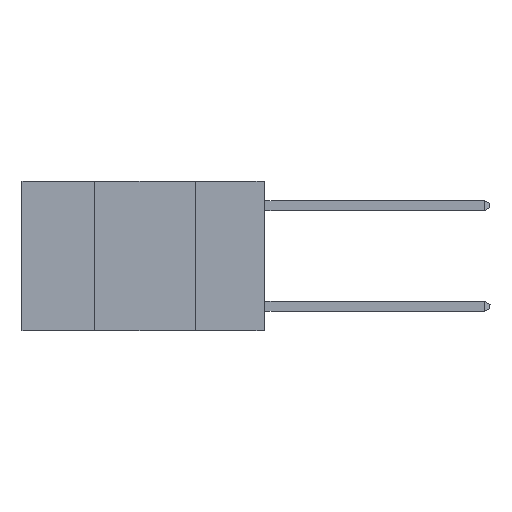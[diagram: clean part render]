
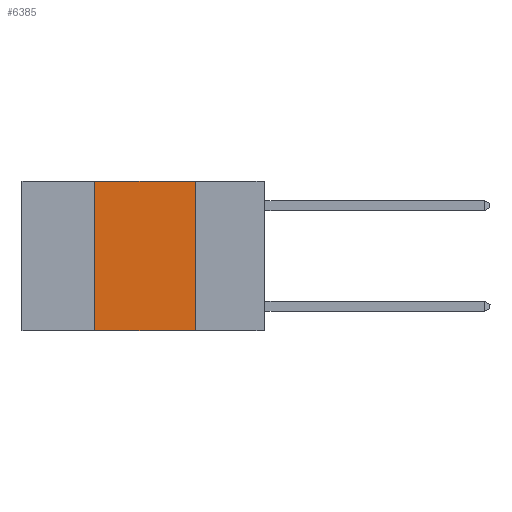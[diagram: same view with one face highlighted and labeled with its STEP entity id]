
A CAD part, left-side view. The second image highlights one B-rep face of the part: STEP entity #6385.
In plain terms, the highlighted planar face has unit normal (-1, 0, 0).
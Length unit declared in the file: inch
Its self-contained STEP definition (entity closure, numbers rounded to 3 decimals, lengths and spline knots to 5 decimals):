
#307 = VECTOR ( 'NONE', #6357, 39.37008 ) ;
#626 = PLANE ( 'NONE',  #1616 ) ;
#719 = LINE ( 'NONE', #3671, #14785 ) ;
#1616 = AXIS2_PLACEMENT_3D ( 'NONE', #10398, #2004, #11815 ) ;
#1763 = CARTESIAN_POINT ( 'NONE',  ( 0., 0.17, 0. ) ) ;
#1870 = VERTEX_POINT ( 'NONE', #9397 ) ;
#2004 = DIRECTION ( 'NONE',  ( 1., 0., 0. ) ) ;
#2241 = DIRECTION ( 'NONE',  ( 0., -1., 0. ) ) ;
#2290 = ORIENTED_EDGE ( 'NONE', *, *, #3329, .F. ) ;
#3329 = EDGE_CURVE ( 'NONE', #8819, #15139, #15619, .T. ) ;
#3671 = CARTESIAN_POINT ( 'NONE',  ( 0., 0.6, 0. ) ) ;
#5928 = LINE ( 'NONE', #17864, #10554 ) ;
#6357 = DIRECTION ( 'NONE',  ( 0., 0., 1. ) ) ;
#6385 = ADVANCED_FACE ( 'NONE', ( #9240 ), #626, .F. ) ;
#8181 = CARTESIAN_POINT ( 'NONE',  ( 0., 0.17, -0.37 ) ) ;
#8328 = ORIENTED_EDGE ( 'NONE', *, *, #16132, .F. ) ;
#8352 = EDGE_CURVE ( 'NONE', #14518, #8819, #719, .T. ) ;
#8451 = EDGE_CURVE ( 'NONE', #1870, #15139, #5928, .T. ) ;
#8819 = VERTEX_POINT ( 'NONE', #1763 ) ;
#9240 = FACE_OUTER_BOUND ( 'NONE', #16139, .T. ) ;
#9397 = CARTESIAN_POINT ( 'NONE',  ( 0., 0.42, -0.37 ) ) ;
#10398 = CARTESIAN_POINT ( 'NONE',  ( 0., 0.6, 0. ) ) ;
#10554 = VECTOR ( 'NONE', #10757, 39.37008 ) ;
#10757 = DIRECTION ( 'NONE',  ( 0., -1., 0. ) ) ;
#10891 = DIRECTION ( 'NONE',  ( 0., 0., -1. ) ) ;
#11191 = ORIENTED_EDGE ( 'NONE', *, *, #8451, .T. ) ;
#11454 = LINE ( 'NONE', #13420, #307 ) ;
#11815 = DIRECTION ( 'NONE',  ( 0., 0., -1. ) ) ;
#11825 = VECTOR ( 'NONE', #10891, 39.37008 ) ;
#13420 = CARTESIAN_POINT ( 'NONE',  ( 0., 0.42, 0. ) ) ;
#14275 = CARTESIAN_POINT ( 'NONE',  ( 0., 0.42, 0. ) ) ;
#14518 = VERTEX_POINT ( 'NONE', #14275 ) ;
#14785 = VECTOR ( 'NONE', #2241, 39.37008 ) ;
#15139 = VERTEX_POINT ( 'NONE', #8181 ) ;
#15619 = LINE ( 'NONE', #18007, #11825 ) ;
#16132 = EDGE_CURVE ( 'NONE', #1870, #14518, #11454, .T. ) ;
#16139 = EDGE_LOOP ( 'NONE', ( #2290, #17302, #8328, #11191 ) ) ;
#17302 = ORIENTED_EDGE ( 'NONE', *, *, #8352, .F. ) ;
#17864 = CARTESIAN_POINT ( 'NONE',  ( 0., 0.6, -0.37 ) ) ;
#18007 = CARTESIAN_POINT ( 'NONE',  ( 0., 0.17, 0. ) ) ;
